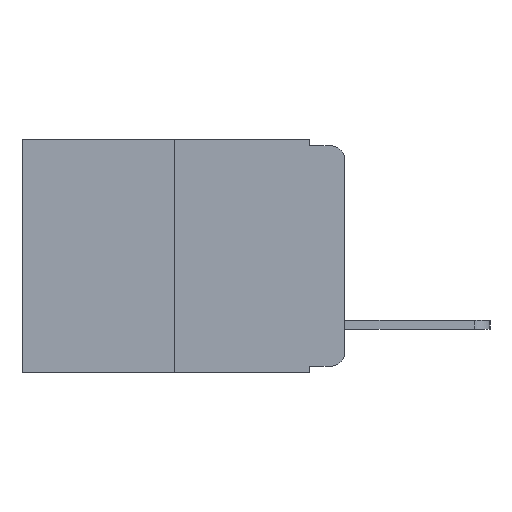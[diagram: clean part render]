
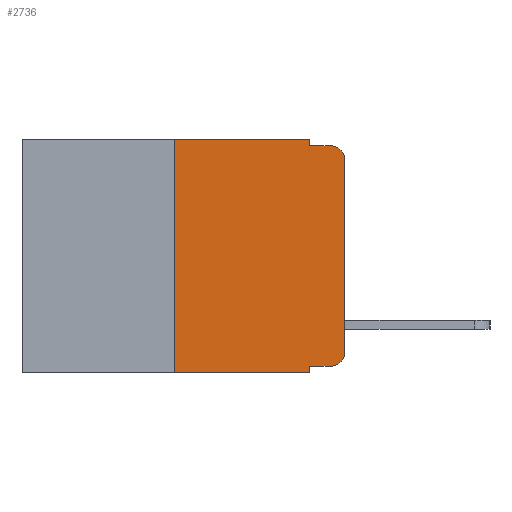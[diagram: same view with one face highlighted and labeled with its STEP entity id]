
A CAD part, left-side view. The second image highlights one B-rep face of the part: STEP entity #2736.
In plain terms, the highlighted planar face has unit normal (-1, 0, 0).
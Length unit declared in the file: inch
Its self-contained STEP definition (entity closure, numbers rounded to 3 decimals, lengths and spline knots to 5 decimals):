
#118 = VERTEX_POINT ( 'NONE', #8285 ) ;
#140 = DIRECTION ( 'NONE',  ( 0., 0., -1. ) ) ;
#209 = ORIENTED_EDGE ( 'NONE', *, *, #11671, .T. ) ;
#459 = ORIENTED_EDGE ( 'NONE', *, *, #11589, .F. ) ;
#499 = VERTEX_POINT ( 'NONE', #7421 ) ;
#757 = CARTESIAN_POINT ( 'NONE',  ( 0., 0.02, -0.313 ) ) ;
#946 = ORIENTED_EDGE ( 'NONE', *, *, #10434, .T. ) ;
#1093 = CARTESIAN_POINT ( 'NONE',  ( 0., 0.02, -0.01 ) ) ;
#1180 = ORIENTED_EDGE ( 'NONE', *, *, #10198, .F. ) ;
#1320 = DIRECTION ( 'NONE',  ( 0., -1., 0. ) ) ;
#1610 = ORIENTED_EDGE ( 'NONE', *, *, #12319, .T. ) ;
#1635 = VECTOR ( 'NONE', #8336, 39.37008 ) ;
#1930 = CARTESIAN_POINT ( 'NONE',  ( 0., 0.25, 0. ) ) ;
#1942 = DIRECTION ( 'NONE',  ( 0., 0., -1. ) ) ;
#1983 = VERTEX_POINT ( 'NONE', #6973 ) ;
#1994 = VERTEX_POINT ( 'NONE', #10766 ) ;
#2216 = EDGE_LOOP ( 'NONE', ( #9073, #9256, #11092, #11774, #459, #1180, #1610, #6888, #946, #209 ) ) ;
#2675 = VECTOR ( 'NONE', #1320, 39.37008 ) ;
#2736 = ADVANCED_FACE ( 'NONE', ( #11741 ), #5361, .F. ) ;
#2787 = VERTEX_POINT ( 'NONE', #3870 ) ;
#2955 = AXIS2_PLACEMENT_3D ( 'NONE', #12248, #6789, #140 ) ;
#2992 = CARTESIAN_POINT ( 'NONE',  ( 0., 0., -0.03 ) ) ;
#3061 = VERTEX_POINT ( 'NONE', #9329 ) ;
#3257 = CIRCLE ( 'NONE', #2955, 0.02 ) ;
#3614 = VECTOR ( 'NONE', #10527, 39.37008 ) ;
#3870 = CARTESIAN_POINT ( 'NONE',  ( 0., 0.051, -0.333 ) ) ;
#4279 = LINE ( 'NONE', #1930, #1635 ) ;
#4324 = CARTESIAN_POINT ( 'NONE',  ( 0., 0.051, 0. ) ) ;
#5080 = CIRCLE ( 'NONE', #8711, 0.02 ) ;
#5103 = CARTESIAN_POINT ( 'NONE',  ( 0., 0.473, 0. ) ) ;
#5132 = DIRECTION ( 'NONE',  ( 0., 0., -1. ) ) ;
#5361 = PLANE ( 'NONE',  #9830 ) ;
#5367 = VERTEX_POINT ( 'NONE', #11881 ) ;
#5423 = VECTOR ( 'NONE', #10059, 39.37008 ) ;
#5435 = DIRECTION ( 'NONE',  ( 1., 0., 0. ) ) ;
#5556 = CARTESIAN_POINT ( 'NONE',  ( 0., 0.051, -0.333 ) ) ;
#5738 = CARTESIAN_POINT ( 'NONE',  ( 0., 0.473, -0.343 ) ) ;
#5754 = LINE ( 'NONE', #5103, #5423 ) ;
#6041 = VERTEX_POINT ( 'NONE', #1093 ) ;
#6083 = CARTESIAN_POINT ( 'NONE',  ( 0., 0.051, -0.01 ) ) ;
#6777 = LINE ( 'NONE', #12143, #3614 ) ;
#6789 = DIRECTION ( 'NONE',  ( -1., 0., 0. ) ) ;
#6888 = ORIENTED_EDGE ( 'NONE', *, *, #10364, .F. ) ;
#6973 = CARTESIAN_POINT ( 'NONE',  ( 0., 0.051, 0. ) ) ;
#7152 = DIRECTION ( 'NONE',  ( 0., -1., 0. ) ) ;
#7261 = CARTESIAN_POINT ( 'NONE',  ( 0., 0.473, 0. ) ) ;
#7421 = CARTESIAN_POINT ( 'NONE',  ( 0., 0.25, -0.343 ) ) ;
#8207 = LINE ( 'NONE', #4324, #12312 ) ;
#8241 = CARTESIAN_POINT ( 'NONE',  ( 0., 0.02, -0.333 ) ) ;
#8285 = CARTESIAN_POINT ( 'NONE',  ( 0., 0.25, 0. ) ) ;
#8336 = DIRECTION ( 'NONE',  ( 0., 0., 1. ) ) ;
#8347 = DIRECTION ( 'NONE',  ( -1., 0., 0. ) ) ;
#8601 = VERTEX_POINT ( 'NONE', #8241 ) ;
#8711 = AXIS2_PLACEMENT_3D ( 'NONE', #757, #8347, #1942 ) ;
#8822 = DIRECTION ( 'NONE',  ( 0., 0., -1. ) ) ;
#8866 = LINE ( 'NONE', #5738, #2675 ) ;
#9073 = ORIENTED_EDGE ( 'NONE', *, *, #9680, .T. ) ;
#9256 = ORIENTED_EDGE ( 'NONE', *, *, #9736, .T. ) ;
#9329 = CARTESIAN_POINT ( 'NONE',  ( 0., 0., -0.313 ) ) ;
#9680 = EDGE_CURVE ( 'NONE', #3061, #11645, #6777, .T. ) ;
#9736 = EDGE_CURVE ( 'NONE', #11645, #6041, #3257, .T. ) ;
#9830 = AXIS2_PLACEMENT_3D ( 'NONE', #7261, #5435, #8822 ) ;
#10059 = DIRECTION ( 'NONE',  ( 0., -1., 0. ) ) ;
#10071 = EDGE_CURVE ( 'NONE', #1994, #6041, #12961, .T. ) ;
#10133 = EDGE_CURVE ( 'NONE', #1983, #1994, #10239, .T. ) ;
#10198 = EDGE_CURVE ( 'NONE', #499, #118, #4279, .T. ) ;
#10239 = LINE ( 'NONE', #12607, #12200 ) ;
#10360 = DIRECTION ( 'NONE',  ( 0., 0., -1. ) ) ;
#10364 = EDGE_CURVE ( 'NONE', #2787, #5367, #8207, .T. ) ;
#10434 = EDGE_CURVE ( 'NONE', #2787, #8601, #11786, .T. ) ;
#10440 = DIRECTION ( 'NONE',  ( 0., -1., 0. ) ) ;
#10527 = DIRECTION ( 'NONE',  ( 0., 0., 1. ) ) ;
#10766 = CARTESIAN_POINT ( 'NONE',  ( 0., 0.051, -0.01 ) ) ;
#11092 = ORIENTED_EDGE ( 'NONE', *, *, #10071, .F. ) ;
#11532 = VECTOR ( 'NONE', #10440, 39.37008 ) ;
#11589 = EDGE_CURVE ( 'NONE', #118, #1983, #5754, .T. ) ;
#11645 = VERTEX_POINT ( 'NONE', #2992 ) ;
#11671 = EDGE_CURVE ( 'NONE', #8601, #3061, #5080, .T. ) ;
#11741 = FACE_OUTER_BOUND ( 'NONE', #2216, .T. ) ;
#11774 = ORIENTED_EDGE ( 'NONE', *, *, #10133, .F. ) ;
#11786 = LINE ( 'NONE', #5556, #11532 ) ;
#11881 = CARTESIAN_POINT ( 'NONE',  ( 0., 0.051, -0.343 ) ) ;
#12143 = CARTESIAN_POINT ( 'NONE',  ( 0., 0., 0. ) ) ;
#12200 = VECTOR ( 'NONE', #5132, 39.37008 ) ;
#12248 = CARTESIAN_POINT ( 'NONE',  ( 0., 0.02, -0.03 ) ) ;
#12312 = VECTOR ( 'NONE', #10360, 39.37008 ) ;
#12319 = EDGE_CURVE ( 'NONE', #499, #5367, #8866, .T. ) ;
#12607 = CARTESIAN_POINT ( 'NONE',  ( 0., 0.051, 0. ) ) ;
#12712 = VECTOR ( 'NONE', #7152, 39.37008 ) ;
#12961 = LINE ( 'NONE', #6083, #12712 ) ;
